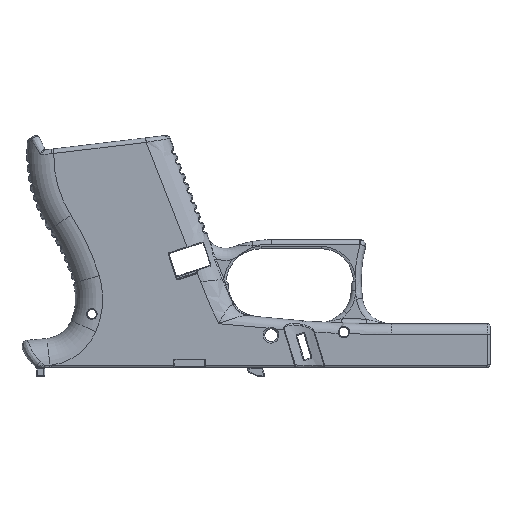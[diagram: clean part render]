
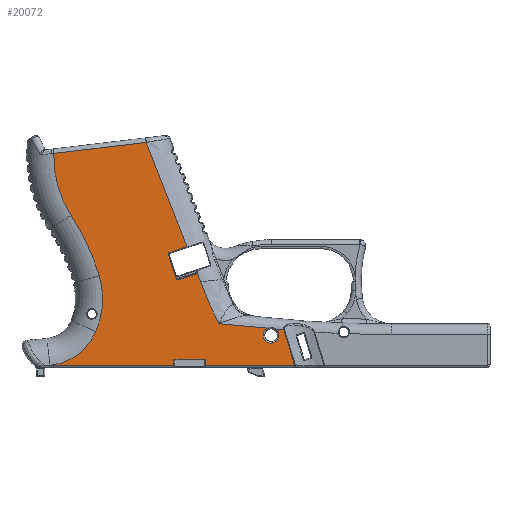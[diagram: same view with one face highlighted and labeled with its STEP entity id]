
A CAD part, front view. The second image highlights one B-rep face of the part: STEP entity #20072.
In plain terms, the highlighted planar face has unit normal (0, -1, 0).
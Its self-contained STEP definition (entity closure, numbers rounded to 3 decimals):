
#1591=FACE_OUTER_BOUND('',#2912,.T.);
#2912=EDGE_LOOP('',(#13993,#13994,#13995,#13996,#13997,#13998,#13999,#14000,
#14001,#14002,#14003,#14004,#14005,#14006,#14007,#14008,#14009,#14010,#14011,
#14012,#14013,#14014,#14015,#14016,#14017,#14018,#14019,#14020));
#4246=CIRCLE('',#21547,0.8);
#4251=CIRCLE('',#21560,2.625);
#4252=CIRCLE('',#21561,2.625);
#4253=CIRCLE('',#21562,156.771);
#4254=CIRCLE('',#21563,0.49);
#4255=CIRCLE('',#21564,0.49);
#4256=CIRCLE('',#21565,0.49);
#4257=CIRCLE('',#21566,35.645);
#4258=CIRCLE('',#21567,77.599);
#4259=CIRCLE('',#21568,27.167);
#4260=CIRCLE('',#21569,18.891);
#6176=LINE('',#32230,#7233);
#6177=LINE('',#32232,#7234);
#6178=LINE('',#32266,#7235);
#6186=LINE('',#32319,#7243);
#6187=LINE('',#32326,#7244);
#6188=LINE('',#32328,#7245);
#6189=LINE('',#32330,#7246);
#6190=LINE('',#32332,#7247);
#6191=LINE('',#32338,#7248);
#6192=LINE('',#32342,#7249);
#6193=LINE('',#32346,#7250);
#6194=LINE('',#32350,#7251);
#6195=LINE('',#32354,#7252);
#6196=LINE('',#32356,#7253);
#6197=LINE('',#32358,#7254);
#6198=LINE('',#32368,#7255);
#6199=LINE('',#32369,#7256);
#7233=VECTOR('',#24389,10.);
#7234=VECTOR('',#24392,10.);
#7235=VECTOR('',#24397,10.);
#7243=VECTOR('',#24425,10.);
#7244=VECTOR('',#24436,10.);
#7245=VECTOR('',#24437,10.);
#7246=VECTOR('',#24438,10.);
#7247=VECTOR('',#24439,10.);
#7248=VECTOR('',#24444,10.);
#7249=VECTOR('',#24447,10.);
#7250=VECTOR('',#24450,10.);
#7251=VECTOR('',#24453,10.);
#7252=VECTOR('',#24456,10.);
#7253=VECTOR('',#24457,10.);
#7254=VECTOR('',#24458,10.);
#7255=VECTOR('',#24467,10.);
#7256=VECTOR('',#24468,10.);
#8430=VERTEX_POINT('',#31881);
#8452=VERTEX_POINT('',#32050);
#8468=VERTEX_POINT('',#32228);
#8469=VERTEX_POINT('',#32257);
#8471=VERTEX_POINT('',#32295);
#8479=VERTEX_POINT('',#32317);
#8480=VERTEX_POINT('',#32325);
#8481=VERTEX_POINT('',#32327);
#8482=VERTEX_POINT('',#32329);
#8483=VERTEX_POINT('',#32331);
#8484=VERTEX_POINT('',#32333);
#8485=VERTEX_POINT('',#32335);
#8486=VERTEX_POINT('',#32337);
#8487=VERTEX_POINT('',#32339);
#8488=VERTEX_POINT('',#32341);
#8489=VERTEX_POINT('',#32343);
#8490=VERTEX_POINT('',#32345);
#8491=VERTEX_POINT('',#32347);
#8492=VERTEX_POINT('',#32349);
#8493=VERTEX_POINT('',#32351);
#8494=VERTEX_POINT('',#32353);
#8495=VERTEX_POINT('',#32355);
#8496=VERTEX_POINT('',#32357);
#8497=VERTEX_POINT('',#32359);
#8498=VERTEX_POINT('',#32361);
#8499=VERTEX_POINT('',#32363);
#8500=VERTEX_POINT('',#32365);
#8501=VERTEX_POINT('',#32367);
#10495=EDGE_CURVE('',#8468,#8430,#6176,.T.);
#10496=EDGE_CURVE('',#8430,#8452,#6177,.T.);
#10499=EDGE_CURVE('',#8452,#8469,#6178,.T.);
#10502=EDGE_CURVE('',#8469,#8471,#4246,.T.);
#10514=EDGE_CURVE('',#8479,#8468,#6186,.T.);
#10517=EDGE_CURVE('',#8480,#8479,#6187,.T.);
#10518=EDGE_CURVE('',#8481,#8480,#6188,.T.);
#10519=EDGE_CURVE('',#8482,#8481,#6189,.T.);
#10520=EDGE_CURVE('',#8483,#8482,#6190,.T.);
#10521=EDGE_CURVE('',#8484,#8483,#4251,.T.);
#10522=EDGE_CURVE('',#8485,#8484,#4252,.T.);
#10523=EDGE_CURVE('',#8486,#8485,#6191,.T.);
#10524=EDGE_CURVE('',#8487,#8486,#4253,.T.);
#10525=EDGE_CURVE('',#8487,#8488,#6192,.T.);
#10526=EDGE_CURVE('',#8489,#8488,#4254,.T.);
#10527=EDGE_CURVE('',#8490,#8489,#6193,.T.);
#10528=EDGE_CURVE('',#8491,#8490,#4255,.T.);
#10529=EDGE_CURVE('',#8492,#8491,#6194,.T.);
#10530=EDGE_CURVE('',#8493,#8492,#4256,.T.);
#10531=EDGE_CURVE('',#8494,#8493,#6195,.T.);
#10532=EDGE_CURVE('',#8494,#8495,#6196,.T.);
#10533=EDGE_CURVE('',#8496,#8495,#6197,.T.);
#10534=EDGE_CURVE('',#8497,#8496,#4257,.T.);
#10535=EDGE_CURVE('',#8498,#8497,#4258,.T.);
#10536=EDGE_CURVE('',#8499,#8498,#4259,.T.);
#10537=EDGE_CURVE('',#8500,#8499,#4260,.T.);
#10538=EDGE_CURVE('',#8501,#8500,#6198,.T.);
#10539=EDGE_CURVE('',#8471,#8501,#6199,.T.);
#13993=ORIENTED_EDGE('',*,*,#10495,.F.);
#13994=ORIENTED_EDGE('',*,*,#10514,.F.);
#13995=ORIENTED_EDGE('',*,*,#10517,.F.);
#13996=ORIENTED_EDGE('',*,*,#10518,.F.);
#13997=ORIENTED_EDGE('',*,*,#10519,.F.);
#13998=ORIENTED_EDGE('',*,*,#10520,.F.);
#13999=ORIENTED_EDGE('',*,*,#10521,.F.);
#14000=ORIENTED_EDGE('',*,*,#10522,.F.);
#14001=ORIENTED_EDGE('',*,*,#10523,.F.);
#14002=ORIENTED_EDGE('',*,*,#10524,.F.);
#14003=ORIENTED_EDGE('',*,*,#10525,.T.);
#14004=ORIENTED_EDGE('',*,*,#10526,.F.);
#14005=ORIENTED_EDGE('',*,*,#10527,.F.);
#14006=ORIENTED_EDGE('',*,*,#10528,.F.);
#14007=ORIENTED_EDGE('',*,*,#10529,.F.);
#14008=ORIENTED_EDGE('',*,*,#10530,.F.);
#14009=ORIENTED_EDGE('',*,*,#10531,.F.);
#14010=ORIENTED_EDGE('',*,*,#10532,.T.);
#14011=ORIENTED_EDGE('',*,*,#10533,.F.);
#14012=ORIENTED_EDGE('',*,*,#10534,.F.);
#14013=ORIENTED_EDGE('',*,*,#10535,.F.);
#14014=ORIENTED_EDGE('',*,*,#10536,.F.);
#14015=ORIENTED_EDGE('',*,*,#10537,.F.);
#14016=ORIENTED_EDGE('',*,*,#10538,.F.);
#14017=ORIENTED_EDGE('',*,*,#10539,.F.);
#14018=ORIENTED_EDGE('',*,*,#10502,.F.);
#14019=ORIENTED_EDGE('',*,*,#10499,.F.);
#14020=ORIENTED_EDGE('',*,*,#10496,.F.);
#19752=PLANE('',#21559);
#20072=ADVANCED_FACE('',(#1591),#19752,.F.);
#21547=AXIS2_PLACEMENT_3D('',#32296,#24402,#24403);
#21559=AXIS2_PLACEMENT_3D('',#32324,#24434,#24435);
#21560=AXIS2_PLACEMENT_3D('',#32334,#24440,#24441);
#21561=AXIS2_PLACEMENT_3D('',#32336,#24442,#24443);
#21562=AXIS2_PLACEMENT_3D('',#32340,#24445,#24446);
#21563=AXIS2_PLACEMENT_3D('',#32344,#24448,#24449);
#21564=AXIS2_PLACEMENT_3D('',#32348,#24451,#24452);
#21565=AXIS2_PLACEMENT_3D('',#32352,#24454,#24455);
#21566=AXIS2_PLACEMENT_3D('',#32360,#24459,#24460);
#21567=AXIS2_PLACEMENT_3D('',#32362,#24461,#24462);
#21568=AXIS2_PLACEMENT_3D('',#32364,#24463,#24464);
#21569=AXIS2_PLACEMENT_3D('',#32366,#24465,#24466);
#24389=DIRECTION('',(0.,0.,1.));
#24392=DIRECTION('',(-1.,0.,0.));
#24397=DIRECTION('',(0.,0.,-1.));
#24402=DIRECTION('center_axis',(0.,-1.,0.));
#24403=DIRECTION('ref_axis',(-0.707,0.,0.707));
#24425=DIRECTION('',(-1.,0.,0.));
#24434=DIRECTION('center_axis',(0.,1.,0.));
#24435=DIRECTION('ref_axis',(1.,0.,0.));
#24436=DIRECTION('',(0.,0.,1.));
#24437=DIRECTION('',(-1.,0.,0.));
#24438=DIRECTION('',(0.292,0.,-0.956));
#24439=DIRECTION('',(0.996,0.,-0.092));
#24440=DIRECTION('center_axis',(0.,-1.,0.));
#24441=DIRECTION('ref_axis',(-1.,0.,0.));
#24442=DIRECTION('center_axis',(0.,-1.,0.));
#24443=DIRECTION('ref_axis',(-1.,0.,0.));
#24444=DIRECTION('',(0.996,0.,-0.092));
#24445=DIRECTION('center_axis',(0.,-1.,0.));
#24446=DIRECTION('ref_axis',(-0.937,0.,-0.35));
#24447=DIRECTION('',(-0.363,0.,0.932));
#24448=DIRECTION('center_axis',(0.,-1.,0.));
#24449=DIRECTION('ref_axis',(0.891,0.,-0.454));
#24450=DIRECTION('',(0.951,0.,0.309));
#24451=DIRECTION('center_axis',(0.,-1.,0.));
#24452=DIRECTION('ref_axis',(-0.454,0.,-0.891));
#24453=DIRECTION('',(0.309,0.,-0.951));
#24454=DIRECTION('center_axis',(0.,-1.,0.));
#24455=DIRECTION('ref_axis',(-0.891,0.,0.454));
#24456=DIRECTION('',(-0.951,0.,-0.309));
#24457=DIRECTION('',(-0.363,0.,0.932));
#24458=DIRECTION('',(0.993,0.,0.119));
#24459=DIRECTION('center_axis',(0.,1.,0.));
#24460=DIRECTION('ref_axis',(-0.961,0.,-0.276));
#24461=DIRECTION('center_axis',(0.,-1.,0.));
#24462=DIRECTION('ref_axis',(0.907,0.,0.421));
#24463=DIRECTION('center_axis',(0.,-1.,0.));
#24464=DIRECTION('ref_axis',(0.998,0.,-0.06));
#24465=DIRECTION('center_axis',(0.,-1.,0.));
#24466=DIRECTION('ref_axis',(0.592,0.,-0.806));
#24467=DIRECTION('',(-1.,0.,0.));
#24468=DIRECTION('',(0.,0.,-1.));
#31881=CARTESIAN_POINT('',(-18.52,-11.5,-23.745));
#32050=CARTESIAN_POINT('',(-28.98,-11.5,-23.745));
#32228=CARTESIAN_POINT('',(-18.52,-11.5,-24.675));
#32230=CARTESIAN_POINT('',(-18.52,-11.5,-7.056));
#32232=CARTESIAN_POINT('',(-10.264,-11.5,-23.745));
#32257=CARTESIAN_POINT('',(-28.98,-11.5,-25.148));
#32266=CARTESIAN_POINT('',(-28.98,-11.5,-7.056));
#32295=CARTESIAN_POINT('',(-29.05,-11.5,-25.475));
#32296=CARTESIAN_POINT('Origin',(-28.25,-11.5,-25.475));
#32317=CARTESIAN_POINT('',(-18.45,-11.5,-24.675));
#32319=CARTESIAN_POINT('',(-10.264,-11.5,-24.675));
#32324=CARTESIAN_POINT('Origin',(-1.777,-11.5,10.863));
#32325=CARTESIAN_POINT('',(-18.45,-11.5,-25.75));
#32326=CARTESIAN_POINT('',(-18.45,-11.5,-7.818));
#32327=CARTESIAN_POINT('',(11.185,-11.5,-25.75));
#32328=CARTESIAN_POINT('',(37.236,-11.5,-25.75));
#32329=CARTESIAN_POINT('',(7.57,-11.5,-13.924));
#32330=CARTESIAN_POINT('',(5.553,-11.5,-7.328));
#32331=CARTESIAN_POINT('',(4.906,-11.5,-13.679));
#32332=CARTESIAN_POINT('',(4.861,-11.5,-13.675));
#32333=CARTESIAN_POINT('',(5.968,-11.5,-15.788));
#32334=CARTESIAN_POINT('Origin',(3.343,-11.5,-15.788));
#32335=CARTESIAN_POINT('',(2.19,-11.5,-13.43));
#32336=CARTESIAN_POINT('Origin',(3.343,-11.5,-15.788));
#32337=CARTESIAN_POINT('',(-14.141,-11.5,-11.929));
#32338=CARTESIAN_POINT('',(4.861,-11.5,-13.675));
#32339=CARTESIAN_POINT('',(-20.166,-11.5,2.06));
#32340=CARTESIAN_POINT('Origin',(126.663,-11.5,57.001));
#32341=CARTESIAN_POINT('',(-21.238,-11.5,4.813));
#32342=CARTESIAN_POINT('',(-37.545,-11.5,46.678));
#32343=CARTESIAN_POINT('',(-21.428,-11.5,4.698));
#32344=CARTESIAN_POINT('Origin',(-21.58,-11.5,5.164));
#32345=CARTESIAN_POINT('',(-27.61,-11.5,2.69));
#32346=CARTESIAN_POINT('',(-11.516,-11.5,7.919));
#32347=CARTESIAN_POINT('',(-28.228,-11.5,3.004));
#32348=CARTESIAN_POINT('Origin',(-27.762,-11.5,3.156));
#32349=CARTESIAN_POINT('',(-30.854,-11.5,11.088));
#32350=CARTESIAN_POINT('',(-28.236,-11.5,3.028));
#32351=CARTESIAN_POINT('',(-30.54,-11.5,11.706));
#32352=CARTESIAN_POINT('Origin',(-30.388,-11.5,11.24));
#32353=CARTESIAN_POINT('',(-24.666,-11.5,13.614));
#32354=CARTESIAN_POINT('',(-17.775,-11.5,15.853));
#32355=CARTESIAN_POINT('',(-38.228,-11.5,48.431));
#32356=CARTESIAN_POINT('',(-37.545,-11.5,46.678));
#32357=CARTESIAN_POINT('',(-68.991,-11.5,44.75));
#32358=CARTESIAN_POINT('',(-18.413,-11.5,50.802));
#32359=CARTESIAN_POINT('',(-63.213,-11.5,24.169));
#32360=CARTESIAN_POINT('Origin',(-33.363,-11.5,43.651));
#32361=CARTESIAN_POINT('',(-53.881,-11.5,4.09));
#32362=CARTESIAN_POINT('Origin',(-128.196,-11.5,-18.243));
#32363=CARTESIAN_POINT('',(-55.002,-11.5,-14.602));
#32364=CARTESIAN_POINT('Origin',(-79.899,-11.5,-3.729));
#32365=CARTESIAN_POINT('',(-69.695,-11.5,-25.75));
#32366=CARTESIAN_POINT('Origin',(-72.315,-11.5,-7.041));
#32367=CARTESIAN_POINT('',(-29.05,-11.5,-25.75));
#32368=CARTESIAN_POINT('',(37.236,-11.5,-25.75));
#32369=CARTESIAN_POINT('',(-29.05,-11.5,-7.056));
